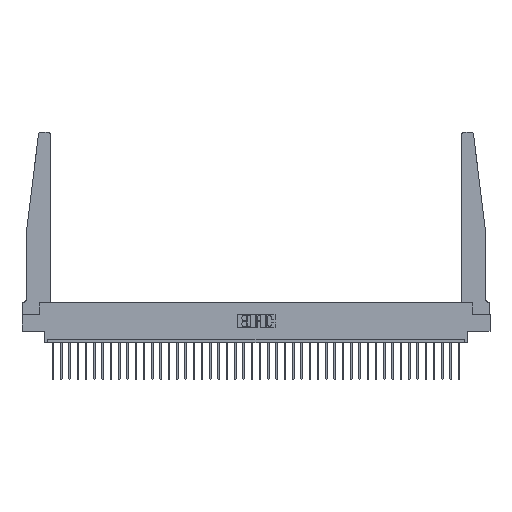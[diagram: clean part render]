
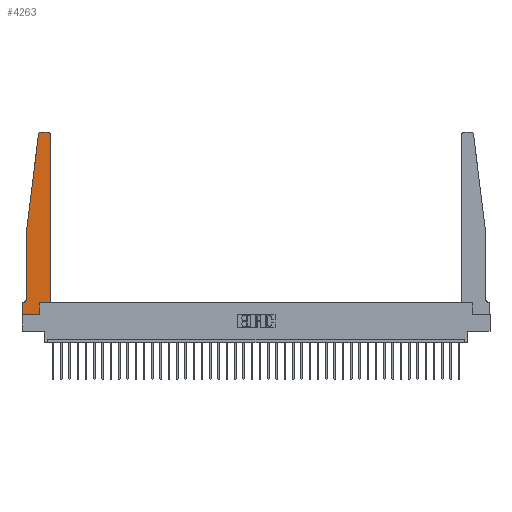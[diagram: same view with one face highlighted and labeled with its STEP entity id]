
A CAD part, top view. The second image highlights one B-rep face of the part: STEP entity #4263.
In plain terms, the highlighted planar face has unit normal (0, 0, 1).
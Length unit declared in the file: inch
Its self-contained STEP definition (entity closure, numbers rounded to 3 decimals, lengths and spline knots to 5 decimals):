
#401 = CIRCLE ( 'NONE', #3265, 0.03 ) ;
#918 = CARTESIAN_POINT ( 'NONE',  ( 0.27653, 2.75, 0.37 ) ) ;
#1027 = EDGE_CURVE ( 'NONE', #29053, #14694, #19213, .T. ) ;
#1478 = VECTOR ( 'NONE', #17769, 39.37008 ) ;
#1647 = LINE ( 'NONE', #10212, #24708 ) ;
#1866 = VERTEX_POINT ( 'NONE', #9823 ) ;
#2757 = DIRECTION ( 'NONE',  ( 0., 1., 0. ) ) ;
#3199 = CARTESIAN_POINT ( 'NONE',  ( 0.425, 0.18, 0.37 ) ) ;
#3265 = AXIS2_PLACEMENT_3D ( 'NONE', #12870, #15025, #21064 ) ;
#3381 = AXIS2_PLACEMENT_3D ( 'NONE', #19901, #12223, #16881 ) ;
#3507 = VERTEX_POINT ( 'NONE', #18708 ) ;
#3872 = ORIENTED_EDGE ( 'NONE', *, *, #32010, .T. ) ;
#4065 = ORIENTED_EDGE ( 'NONE', *, *, #28080, .T. ) ;
#4113 = ORIENTED_EDGE ( 'NONE', *, *, #22518, .T. ) ;
#4263 = ADVANCED_FACE ( 'NONE', ( #14889 ), #6153, .T. ) ;
#4514 = LINE ( 'NONE', #7200, #13103 ) ;
#6153 = PLANE ( 'NONE',  #3381 ) ;
#6433 = EDGE_CURVE ( 'NONE', #33846, #28533, #8974, .T. ) ;
#6869 = CARTESIAN_POINT ( 'NONE',  ( 0., 0., 0.37 ) ) ;
#7152 = EDGE_LOOP ( 'NONE', ( #3872, #28503, #32308, #9321, #29628, #16427, #29236, #7954, #24984, #4113, #4065, #32719 ) ) ;
#7200 = CARTESIAN_POINT ( 'NONE',  ( 0.25, 2.75, 0.37 ) ) ;
#7632 = DIRECTION ( 'NONE',  ( -1., 0., 0. ) ) ;
#7954 = ORIENTED_EDGE ( 'NONE', *, *, #18008, .T. ) ;
#8113 = VERTEX_POINT ( 'NONE', #25541 ) ;
#8233 = CARTESIAN_POINT ( 'NONE',  ( 0.015, 0.1875, 0.37 ) ) ;
#8346 = LINE ( 'NONE', #35310, #16304 ) ;
#8899 = LINE ( 'NONE', #3199, #18026 ) ;
#8974 = LINE ( 'NONE', #22555, #10875 ) ;
#9130 = EDGE_CURVE ( 'NONE', #8113, #1866, #26854, .T. ) ;
#9321 = ORIENTED_EDGE ( 'NONE', *, *, #13677, .T. ) ;
#9823 = CARTESIAN_POINT ( 'NONE',  ( 0.2605, 0.18, 0.37 ) ) ;
#10135 = DIRECTION ( 'NONE',  ( 0., 0., -1. ) ) ;
#10212 = CARTESIAN_POINT ( 'NONE',  ( 0.425, 0.18, 0.37 ) ) ;
#10875 = VECTOR ( 'NONE', #11485, 39.37008 ) ;
#11295 = VECTOR ( 'NONE', #26333, 39.37008 ) ;
#11485 = DIRECTION ( 'NONE',  ( -1., 0., 0. ) ) ;
#12041 = CARTESIAN_POINT ( 'NONE',  ( 0.425, 0.18, 0.37 ) ) ;
#12205 = DIRECTION ( 'NONE',  ( 1., 0., 0. ) ) ;
#12223 = DIRECTION ( 'NONE',  ( 0., 0., 1. ) ) ;
#12396 = LINE ( 'NONE', #29160, #16485 ) ;
#12841 = CARTESIAN_POINT ( 'NONE',  ( 0.395, 2.75, 0.37 ) ) ;
#12870 = CARTESIAN_POINT ( 'NONE',  ( 0.395, 2.72, 0.37 ) ) ;
#13103 = VECTOR ( 'NONE', #26296, 39.37008 ) ;
#13168 = CARTESIAN_POINT ( 'NONE',  ( 0.015, 0.2375, 0.37 ) ) ;
#13677 = EDGE_CURVE ( 'NONE', #3507, #27355, #8346, .T. ) ;
#14238 = VERTEX_POINT ( 'NONE', #12041 ) ;
#14557 = DIRECTION ( 'NONE',  ( 1., 0., 0. ) ) ;
#14694 = VERTEX_POINT ( 'NONE', #15515 ) ;
#14889 = FACE_OUTER_BOUND ( 'NONE', #7152, .T. ) ;
#15025 = DIRECTION ( 'NONE',  ( 0., 0., 1. ) ) ;
#15069 = CARTESIAN_POINT ( 'NONE',  ( 0., 0.1875, 0.37 ) ) ;
#15515 = CARTESIAN_POINT ( 'NONE',  ( 0.24675, 2.72367, 0.37 ) ) ;
#16304 = VECTOR ( 'NONE', #30131, 39.37008 ) ;
#16427 = ORIENTED_EDGE ( 'NONE', *, *, #6433, .T. ) ;
#16485 = VECTOR ( 'NONE', #28986, 39.37008 ) ;
#16881 = DIRECTION ( 'NONE',  ( 1., 0., 0. ) ) ;
#17769 = DIRECTION ( 'NONE',  ( 0., -1., 0. ) ) ;
#17957 = DIRECTION ( 'NONE',  ( 0., 1., 0. ) ) ;
#18008 = EDGE_CURVE ( 'NONE', #34257, #8113, #12396, .T. ) ;
#18026 = VECTOR ( 'NONE', #17957, 39.37008 ) ;
#18708 = CARTESIAN_POINT ( 'NONE',  ( 0.065, 1.25, 0.37 ) ) ;
#18832 = AXIS2_PLACEMENT_3D ( 'NONE', #13168, #10135, #7632 ) ;
#19192 = CARTESIAN_POINT ( 'NONE',  ( 0.2605, 0.18, 0.37 ) ) ;
#19213 = CIRCLE ( 'NONE', #34034, 0.03 ) ;
#19671 = CARTESIAN_POINT ( 'NONE',  ( 0.425, 2.72, 0.37 ) ) ;
#19846 = VERTEX_POINT ( 'NONE', #12841 ) ;
#19901 = CARTESIAN_POINT ( 'NONE',  ( 0., 0.1875, 0.37 ) ) ;
#20617 = LINE ( 'NONE', #6869, #1478 ) ;
#21064 = DIRECTION ( 'NONE',  ( 1., 0., 0. ) ) ;
#21096 = CARTESIAN_POINT ( 'NONE',  ( 0.065, 0.2375, 0.37 ) ) ;
#22054 = CARTESIAN_POINT ( 'NONE',  ( 0.27653, 2.72, 0.37 ) ) ;
#22518 = EDGE_CURVE ( 'NONE', #1866, #14238, #1647, .T. ) ;
#22555 = CARTESIAN_POINT ( 'NONE',  ( 0.065, 0.1875, 0.37 ) ) ;
#22797 = VERTEX_POINT ( 'NONE', #19671 ) ;
#24708 = VECTOR ( 'NONE', #12205, 39.37008 ) ;
#24984 = ORIENTED_EDGE ( 'NONE', *, *, #9130, .T. ) ;
#25541 = CARTESIAN_POINT ( 'NONE',  ( 0.2605, 0., 0.37 ) ) ;
#25789 = EDGE_CURVE ( 'NONE', #28533, #34257, #20617, .T. ) ;
#26296 = DIRECTION ( 'NONE',  ( -1., 0., 0. ) ) ;
#26333 = DIRECTION ( 'NONE',  ( -0.122, -0.992, 0. ) ) ;
#26854 = LINE ( 'NONE', #19192, #28614 ) ;
#27355 = VERTEX_POINT ( 'NONE', #21096 ) ;
#28080 = EDGE_CURVE ( 'NONE', #14238, #22797, #8899, .T. ) ;
#28503 = ORIENTED_EDGE ( 'NONE', *, *, #1027, .T. ) ;
#28533 = VERTEX_POINT ( 'NONE', #15069 ) ;
#28614 = VECTOR ( 'NONE', #2757, 39.37008 ) ;
#28986 = DIRECTION ( 'NONE',  ( 1., 0., 0. ) ) ;
#29053 = VERTEX_POINT ( 'NONE', #918 ) ;
#29160 = CARTESIAN_POINT ( 'NONE',  ( 0., 0., 0.37 ) ) ;
#29211 = EDGE_CURVE ( 'NONE', #22797, #19846, #401, .T. ) ;
#29236 = ORIENTED_EDGE ( 'NONE', *, *, #25789, .T. ) ;
#29628 = ORIENTED_EDGE ( 'NONE', *, *, #33066, .T. ) ;
#30131 = DIRECTION ( 'NONE',  ( 0., -1., 0. ) ) ;
#30182 = EDGE_CURVE ( 'NONE', #14694, #3507, #34017, .T. ) ;
#30812 = CIRCLE ( 'NONE', #18832, 0.05 ) ;
#30965 = DIRECTION ( 'NONE',  ( 0., 0., 1. ) ) ;
#31326 = CARTESIAN_POINT ( 'NONE',  ( 0.065, 1.25, 0.37 ) ) ;
#32010 = EDGE_CURVE ( 'NONE', #19846, #29053, #4514, .T. ) ;
#32308 = ORIENTED_EDGE ( 'NONE', *, *, #30182, .T. ) ;
#32719 = ORIENTED_EDGE ( 'NONE', *, *, #29211, .T. ) ;
#33066 = EDGE_CURVE ( 'NONE', #27355, #33846, #30812, .T. ) ;
#33846 = VERTEX_POINT ( 'NONE', #8233 ) ;
#34017 = LINE ( 'NONE', #31326, #11295 ) ;
#34034 = AXIS2_PLACEMENT_3D ( 'NONE', #22054, #30965, #14557 ) ;
#34257 = VERTEX_POINT ( 'NONE', #35176 ) ;
#35176 = CARTESIAN_POINT ( 'NONE',  ( 0., 0., 0.37 ) ) ;
#35310 = CARTESIAN_POINT ( 'NONE',  ( 0.065, 1.25, 0.37 ) ) ;
